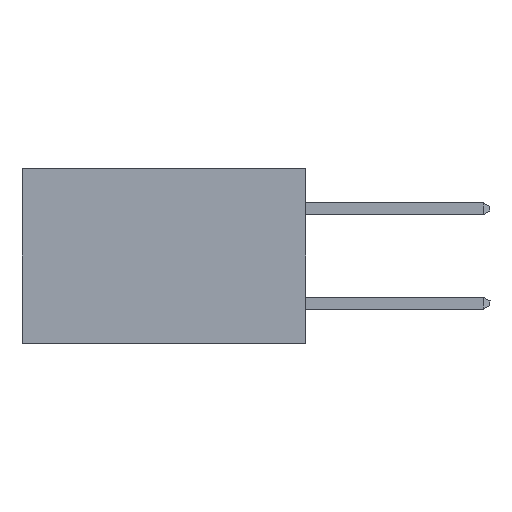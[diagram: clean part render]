
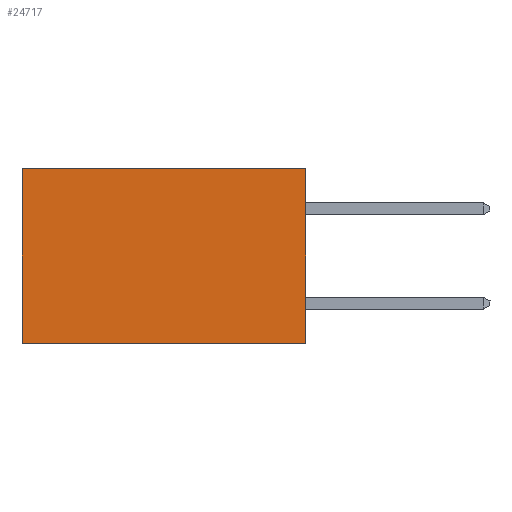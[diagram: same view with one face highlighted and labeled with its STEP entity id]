
A CAD part, left-side view. The second image highlights one B-rep face of the part: STEP entity #24717.
In plain terms, the highlighted planar face has unit normal (-1, 0, 0).
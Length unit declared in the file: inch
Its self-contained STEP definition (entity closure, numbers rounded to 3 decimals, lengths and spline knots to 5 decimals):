
#534 = CARTESIAN_POINT ( 'NONE',  ( 0.298, 0., 0. ) ) ;
#884 = LINE ( 'NONE', #3324, #5763 ) ;
#977 = VECTOR ( 'NONE', #1138, 39.37008 ) ;
#1138 = DIRECTION ( 'NONE',  ( 0., 0., -1. ) ) ;
#1187 = DIRECTION ( 'NONE',  ( 0., 1., 0. ) ) ;
#1325 = VERTEX_POINT ( 'NONE', #2218 ) ;
#1834 = FACE_OUTER_BOUND ( 'NONE', #13011, .T. ) ;
#2065 = CARTESIAN_POINT ( 'NONE',  ( 0.298, 0., -0.37 ) ) ;
#2218 = CARTESIAN_POINT ( 'NONE',  ( 0.298, 0.6, -0.37 ) ) ;
#2422 = EDGE_CURVE ( 'NONE', #14544, #1325, #884, .T. ) ;
#3097 = AXIS2_PLACEMENT_3D ( 'NONE', #5188, #22628, #24709 ) ;
#3217 = PLANE ( 'NONE',  #3097 ) ;
#3324 = CARTESIAN_POINT ( 'NONE',  ( 0.298, 0., -0.37 ) ) ;
#3692 = LINE ( 'NONE', #17033, #24084 ) ;
#5188 = CARTESIAN_POINT ( 'NONE',  ( 0.298, 0., 0. ) ) ;
#5763 = VECTOR ( 'NONE', #1187, 39.37008 ) ;
#6131 = VECTOR ( 'NONE', #16098, 39.37008 ) ;
#6162 = CARTESIAN_POINT ( 'NONE',  ( 0.298, 0.6, 0. ) ) ;
#6660 = VERTEX_POINT ( 'NONE', #6162 ) ;
#7778 = ORIENTED_EDGE ( 'NONE', *, *, #15823, .T. ) ;
#9789 = CARTESIAN_POINT ( 'NONE',  ( 0.298, 0., 0. ) ) ;
#11025 = ORIENTED_EDGE ( 'NONE', *, *, #2422, .F. ) ;
#13011 = EDGE_LOOP ( 'NONE', ( #15967, #11025, #20282, #7778 ) ) ;
#14544 = VERTEX_POINT ( 'NONE', #2065 ) ;
#14977 = EDGE_CURVE ( 'NONE', #16898, #14544, #19874, .T. ) ;
#15823 = EDGE_CURVE ( 'NONE', #16898, #6660, #21953, .T. ) ;
#15967 = ORIENTED_EDGE ( 'NONE', *, *, #21878, .T. ) ;
#16098 = DIRECTION ( 'NONE',  ( 0., 1., 0. ) ) ;
#16898 = VERTEX_POINT ( 'NONE', #9789 ) ;
#17033 = CARTESIAN_POINT ( 'NONE',  ( 0.298, 0.6, 0. ) ) ;
#19874 = LINE ( 'NONE', #24349, #977 ) ;
#20282 = ORIENTED_EDGE ( 'NONE', *, *, #14977, .F. ) ;
#20802 = DIRECTION ( 'NONE',  ( 0., 0., -1. ) ) ;
#21878 = EDGE_CURVE ( 'NONE', #6660, #1325, #3692, .T. ) ;
#21953 = LINE ( 'NONE', #534, #6131 ) ;
#22628 = DIRECTION ( 'NONE',  ( 1., 0., 0. ) ) ;
#24084 = VECTOR ( 'NONE', #20802, 39.37008 ) ;
#24349 = CARTESIAN_POINT ( 'NONE',  ( 0.298, 0., 0. ) ) ;
#24709 = DIRECTION ( 'NONE',  ( 0., 0., -1. ) ) ;
#24717 = ADVANCED_FACE ( 'NONE', ( #1834 ), #3217, .F. ) ;
